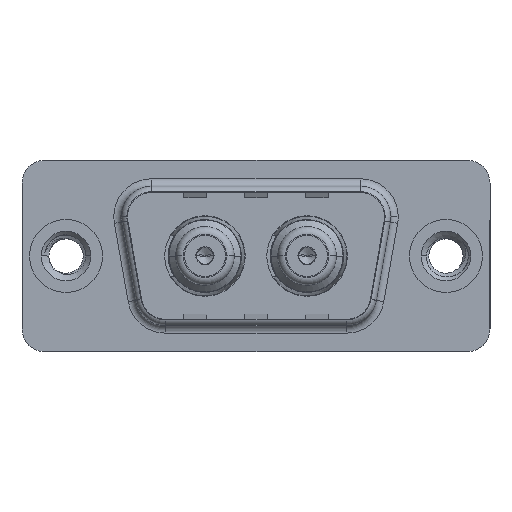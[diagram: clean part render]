
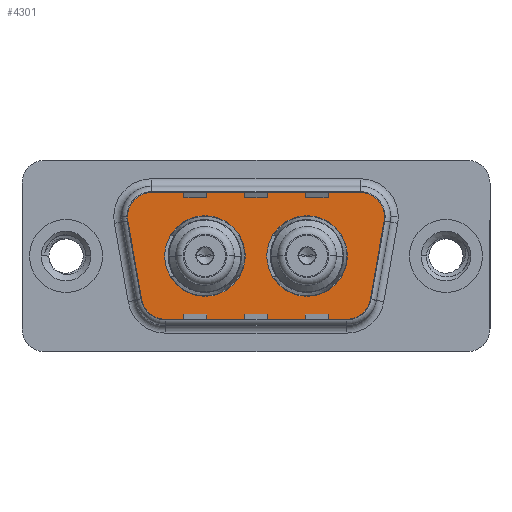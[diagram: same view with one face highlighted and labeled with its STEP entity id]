
A CAD part, top view. The second image highlights one B-rep face of the part: STEP entity #4301.
In plain terms, the highlighted planar face has unit normal (0, 0, 1).
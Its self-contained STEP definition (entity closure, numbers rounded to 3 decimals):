
#2 = CARTESIAN_POINT ( 'NONE',  ( 4.489, -3.247, 0. ) ) ;
#151 = EDGE_CURVE ( 'NONE', #13156, #12910, #1539, .T. ) ;
#1012 = VECTOR ( 'NONE', #8587, 1000. ) ;
#1205 = ORIENTED_EDGE ( 'NONE', *, *, #8679, .T. ) ;
#1278 = VERTEX_POINT ( 'NONE', #11976 ) ;
#1318 = CIRCLE ( 'NONE', #14260, 2.65 ) ;
#1445 = EDGE_CURVE ( 'NONE', #8216, #4203, #7051, .T. ) ;
#1457 = VERTEX_POINT ( 'NONE', #9179 ) ;
#1478 = CARTESIAN_POINT ( 'NONE',  ( 6.49, 0., 0. ) ) ;
#1539 = LINE ( 'NONE', #4401, #15405 ) ;
#1540 = ORIENTED_EDGE ( 'NONE', *, *, #3657, .F. ) ;
#1615 = PLANE ( 'NONE',  #4743 ) ;
#1723 = FACE_BOUND ( 'NONE', #13966, .T. ) ;
#1746 = EDGE_LOOP ( 'NONE', ( #12581, #3810 ) ) ;
#1794 = CIRCLE ( 'NONE', #5109, 2. ) ;
#1925 = CIRCLE ( 'NONE', #14459, 2.65 ) ;
#2244 = ORIENTED_EDGE ( 'NONE', *, *, #5474, .T. ) ;
#2548 = EDGE_CURVE ( 'NONE', #8524, #16319, #9497, .T. ) ;
#2786 = CARTESIAN_POINT ( 'NONE',  ( 5.436, 2.9, 0. ) ) ;
#2929 = ORIENTED_EDGE ( 'NONE', *, *, #14225, .T. ) ;
#3153 = EDGE_CURVE ( 'NONE', #5044, #13504, #16780, .T. ) ;
#3657 = EDGE_CURVE ( 'NONE', #16319, #8524, #1925, .T. ) ;
#3810 = ORIENTED_EDGE ( 'NONE', *, *, #5496, .F. ) ;
#3819 = DIRECTION ( 'NONE',  ( 0., 0., 1. ) ) ;
#3976 = CARTESIAN_POINT ( 'NONE',  ( 15.86, 0., 0. ) ) ;
#4070 = DIRECTION ( 'NONE',  ( 1., 0., 0. ) ) ;
#4072 = AXIS2_PLACEMENT_3D ( 'NONE', #3976, #3819, #10336 ) ;
#4090 = CARTESIAN_POINT ( 'NONE',  ( 18.541, -2.9, 0. ) ) ;
#4203 = VERTEX_POINT ( 'NONE', #6714 ) ;
#4237 = EDGE_LOOP ( 'NONE', ( #12773, #7812, #16461, #15151, #9298, #2929, #8095, #1205, #2244 ) ) ;
#4269 = AXIS2_PLACEMENT_3D ( 'NONE', #7557, #5326, #8728 ) ;
#4289 = CARTESIAN_POINT ( 'NONE',  ( 6.459, -2.9, 0. ) ) ;
#4301 = ADVANCED_FACE ( 'NONE', ( #12135, #1723, #8687 ), #1615, .T. ) ;
#4401 = CARTESIAN_POINT ( 'NONE',  ( 3.466, 2.553, 0. ) ) ;
#4457 = DIRECTION ( 'NONE',  ( -1., 0., 0. ) ) ;
#4743 = AXIS2_PLACEMENT_3D ( 'NONE', #12049, #7739, #7845 ) ;
#4747 = ORIENTED_EDGE ( 'NONE', *, *, #2548, .F. ) ;
#4864 = LINE ( 'NONE', #7247, #1012 ) ;
#4951 = DIRECTION ( 'NONE',  ( 1., 0., 0. ) ) ;
#4969 = EDGE_CURVE ( 'NONE', #14809, #1278, #7415, .T. ) ;
#5044 = VERTEX_POINT ( 'NONE', #13097 ) ;
#5109 = AXIS2_PLACEMENT_3D ( 'NONE', #4289, #13417, #5607 ) ;
#5188 = CARTESIAN_POINT ( 'NONE',  ( 15.86, 0., 0. ) ) ;
#5212 = CARTESIAN_POINT ( 'NONE',  ( 5.436, 4.9, 0. ) ) ;
#5326 = DIRECTION ( 'NONE',  ( 0., 0., 1. ) ) ;
#5412 = DIRECTION ( 'NONE',  ( 1., 0., 0. ) ) ;
#5474 = EDGE_CURVE ( 'NONE', #1457, #12221, #6783, .T. ) ;
#5496 = EDGE_CURVE ( 'NONE', #1278, #14809, #1318, .T. ) ;
#5607 = DIRECTION ( 'NONE',  ( -1., 0., 0. ) ) ;
#5813 = CARTESIAN_POINT ( 'NONE',  ( 9.14, 0., 0. ) ) ;
#5972 = VECTOR ( 'NONE', #12894, 1000. ) ;
#6138 = EDGE_CURVE ( 'NONE', #12221, #15909, #11036, .T. ) ;
#6309 = AXIS2_PLACEMENT_3D ( 'NONE', #4090, #13217, #5412 ) ;
#6408 = DIRECTION ( 'NONE',  ( 0.174, -0.985, 0. ) ) ;
#6467 = CARTESIAN_POINT ( 'NONE',  ( 18.541, -4.9, 0. ) ) ;
#6516 = DIRECTION ( 'NONE',  ( 1., 0., 0. ) ) ;
#6714 = CARTESIAN_POINT ( 'NONE',  ( 5.436, 4.9, 0. ) ) ;
#6783 = LINE ( 'NONE', #7716, #5972 ) ;
#7051 = LINE ( 'NONE', #5212, #16014 ) ;
#7070 = CARTESIAN_POINT ( 'NONE',  ( 19.564, 2.9, 0. ) ) ;
#7247 = CARTESIAN_POINT ( 'NONE',  ( 21.534, 2.553, 0. ) ) ;
#7415 = CIRCLE ( 'NONE', #4072, 2.65 ) ;
#7557 = CARTESIAN_POINT ( 'NONE',  ( 19.564, 2.9, 0. ) ) ;
#7716 = CARTESIAN_POINT ( 'NONE',  ( 6.459, -4.9, 0. ) ) ;
#7739 = DIRECTION ( 'NONE',  ( 0., 0., 1. ) ) ;
#7812 = ORIENTED_EDGE ( 'NONE', *, *, #8177, .T. ) ;
#7845 = DIRECTION ( 'NONE',  ( 1., 0., 0. ) ) ;
#8095 = ORIENTED_EDGE ( 'NONE', *, *, #151, .T. ) ;
#8177 = EDGE_CURVE ( 'NONE', #15909, #5044, #4864, .T. ) ;
#8216 = VERTEX_POINT ( 'NONE', #12568 ) ;
#8403 = DIRECTION ( 'NONE',  ( -1., 0., 0. ) ) ;
#8524 = VERTEX_POINT ( 'NONE', #1478 ) ;
#8587 = DIRECTION ( 'NONE',  ( 0.174, 0.985, 0. ) ) ;
#8679 = EDGE_CURVE ( 'NONE', #12910, #1457, #1794, .T. ) ;
#8687 = FACE_OUTER_BOUND ( 'NONE', #4237, .T. ) ;
#8728 = DIRECTION ( 'NONE',  ( -1., 0., 0. ) ) ;
#9179 = CARTESIAN_POINT ( 'NONE',  ( 6.459, -4.9, 0. ) ) ;
#9298 = ORIENTED_EDGE ( 'NONE', *, *, #1445, .T. ) ;
#9497 = CIRCLE ( 'NONE', #15745, 2.65 ) ;
#9837 = DIRECTION ( 'NONE',  ( 0., 0., 1. ) ) ;
#10302 = CARTESIAN_POINT ( 'NONE',  ( 18.51, 0., 0. ) ) ;
#10336 = DIRECTION ( 'NONE',  ( 1., 0., 0. ) ) ;
#11036 = CIRCLE ( 'NONE', #6309, 2. ) ;
#11141 = CARTESIAN_POINT ( 'NONE',  ( 21.564, 2.9, 0. ) ) ;
#11924 = DIRECTION ( 'NONE',  ( 0., 0., 1. ) ) ;
#11976 = CARTESIAN_POINT ( 'NONE',  ( 13.21, 0., 0. ) ) ;
#12049 = CARTESIAN_POINT ( 'NONE',  ( 18.541, -2.9, 0. ) ) ;
#12135 = FACE_BOUND ( 'NONE', #1746, .T. ) ;
#12221 = VERTEX_POINT ( 'NONE', #6467 ) ;
#12568 = CARTESIAN_POINT ( 'NONE',  ( 19.564, 4.9, 0. ) ) ;
#12581 = ORIENTED_EDGE ( 'NONE', *, *, #4969, .F. ) ;
#12773 = ORIENTED_EDGE ( 'NONE', *, *, #6138, .T. ) ;
#12894 = DIRECTION ( 'NONE',  ( 1., 0., 0. ) ) ;
#12910 = VERTEX_POINT ( 'NONE', #2 ) ;
#13097 = CARTESIAN_POINT ( 'NONE',  ( 21.534, 2.553, 0. ) ) ;
#13156 = VERTEX_POINT ( 'NONE', #14985 ) ;
#13217 = DIRECTION ( 'NONE',  ( 0., 0., 1. ) ) ;
#13417 = DIRECTION ( 'NONE',  ( 0., 0., 1. ) ) ;
#13504 = VERTEX_POINT ( 'NONE', #11141 ) ;
#13567 = CIRCLE ( 'NONE', #16859, 2. ) ;
#13764 = CIRCLE ( 'NONE', #15681, 2. ) ;
#13817 = EDGE_CURVE ( 'NONE', #13504, #8216, #13567, .T. ) ;
#13966 = EDGE_LOOP ( 'NONE', ( #1540, #4747 ) ) ;
#14074 = DIRECTION ( 'NONE',  ( 0., 0., 1. ) ) ;
#14225 = EDGE_CURVE ( 'NONE', #4203, #13156, #13764, .T. ) ;
#14260 = AXIS2_PLACEMENT_3D ( 'NONE', #5188, #14314, #6516 ) ;
#14314 = DIRECTION ( 'NONE',  ( 0., 0., 1. ) ) ;
#14459 = AXIS2_PLACEMENT_3D ( 'NONE', #14587, #14074, #15225 ) ;
#14587 = CARTESIAN_POINT ( 'NONE',  ( 9.14, 0., 0. ) ) ;
#14809 = VERTEX_POINT ( 'NONE', #10302 ) ;
#14985 = CARTESIAN_POINT ( 'NONE',  ( 3.466, 2.553, 0. ) ) ;
#15151 = ORIENTED_EDGE ( 'NONE', *, *, #13817, .T. ) ;
#15225 = DIRECTION ( 'NONE',  ( 1., 0., 0. ) ) ;
#15405 = VECTOR ( 'NONE', #6408, 1000. ) ;
#15681 = AXIS2_PLACEMENT_3D ( 'NONE', #2786, #11924, #4070 ) ;
#15745 = AXIS2_PLACEMENT_3D ( 'NONE', #5813, #9837, #4951 ) ;
#15900 = CARTESIAN_POINT ( 'NONE',  ( 20.511, -3.247, 0. ) ) ;
#15909 = VERTEX_POINT ( 'NONE', #15900 ) ;
#16014 = VECTOR ( 'NONE', #4457, 1000. ) ;
#16155 = DIRECTION ( 'NONE',  ( 0., 0., 1. ) ) ;
#16319 = VERTEX_POINT ( 'NONE', #16586 ) ;
#16461 = ORIENTED_EDGE ( 'NONE', *, *, #3153, .T. ) ;
#16586 = CARTESIAN_POINT ( 'NONE',  ( 11.79, 0., 0. ) ) ;
#16780 = CIRCLE ( 'NONE', #4269, 2. ) ;
#16859 = AXIS2_PLACEMENT_3D ( 'NONE', #7070, #16155, #8403 ) ;
